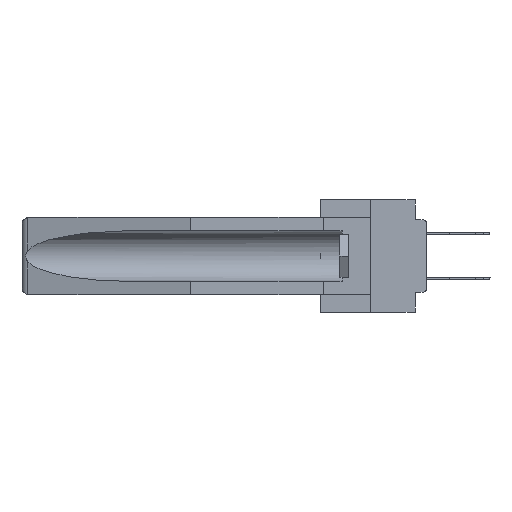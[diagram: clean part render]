
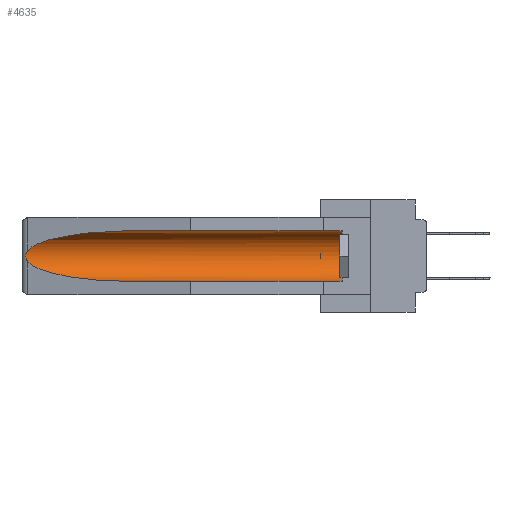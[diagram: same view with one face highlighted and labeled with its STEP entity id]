
A CAD part, left-side view. The second image highlights one B-rep face of the part: STEP entity #4635.
In plain terms, the highlighted cylindrical face has radius 2.857 mm (diameter 5.715 mm), a partial arc.
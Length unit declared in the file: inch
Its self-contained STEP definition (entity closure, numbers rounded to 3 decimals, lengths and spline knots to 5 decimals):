
#343 = VERTEX_POINT ( 'NONE', #15983 ) ;
#2285 = CARTESIAN_POINT ( 'NONE',  ( 0.25451, 1.48313, -0.09465 ) ) ;
#2305 = CARTESIAN_POINT ( 'NONE',  ( 0.155, 0.126, -0.059 ) ) ;
#3150 = CARTESIAN_POINT ( 'NONE',  ( 0.26654, 1.53092, -0.15636 ) ) ;
#3228 = CARTESIAN_POINT ( 'NONE',  ( 0.155, 1.07973, -0.059 ) ) ;
#3517 = VERTEX_POINT ( 'NONE', #33483 ) ;
#4357 = EDGE_LOOP ( 'NONE', ( #16851, #13182, #14924, #16887, #33822, #25248 ) ) ;
#4635 = ADVANCED_FACE ( 'NONE', ( #13232 ), #30506, .F. ) ;
#4799 = EDGE_CURVE ( 'NONE', #22760, #343, #28075, .T. ) ;
#6277 = CARTESIAN_POINT ( 'NONE',  ( 0.2675, 1.53308, -0.16763 ) ) ;
#8865 = DIRECTION ( 'NONE',  ( 0., 1., 0. ) ) ;
#9593 =( BOUNDED_CURVE ( )  B_SPLINE_CURVE ( 3, ( #3228, #29074, #2285, #34038 ),
 .UNSPECIFIED., .F., .F. ) 
 B_SPLINE_CURVE_WITH_KNOTS ( ( 4, 4 ),
 ( 4.71239, 6.08839 ),
 .UNSPECIFIED. ) 
 CURVE ( )  GEOMETRIC_REPRESENTATION_ITEM ( )  RATIONAL_B_SPLINE_CURVE ( ( 1., 0.848, 0.848, 1. ) ) 
 REPRESENTATION_ITEM ( '' )  );
#9688 = CARTESIAN_POINT ( 'NONE',  ( 0.26537, 1.52718, -0.14972 ) ) ;
#10539 = CARTESIAN_POINT ( 'NONE',  ( 0.26537, 1.52718, -0.14972 ) ) ;
#11886 =( BOUNDED_CURVE ( )  B_SPLINE_CURVE ( 3, ( #27432, #27709, #34202, #28121 ),
 .UNSPECIFIED., .F., .T. ) 
 B_SPLINE_CURVE_WITH_KNOTS ( ( 4, 4 ),
 ( 0.1948, 1.5708 ),
 .UNSPECIFIED. ) 
 CURVE ( )  GEOMETRIC_REPRESENTATION_ITEM ( )  RATIONAL_B_SPLINE_CURVE ( ( 1., 0.848, 0.848, 1. ) ) 
 REPRESENTATION_ITEM ( '' )  );
#12557 = CARTESIAN_POINT ( 'NONE',  ( 0.155, 0.126, -0.1715 ) ) ;
#13182 = ORIENTED_EDGE ( 'NONE', *, *, #37447, .T. ) ;
#13232 = FACE_OUTER_BOUND ( 'NONE', #4357, .T. ) ;
#13719 = LINE ( 'NONE', #17960, #37736 ) ;
#14924 = ORIENTED_EDGE ( 'NONE', *, *, #31422, .T. ) ;
#15839 = DIRECTION ( 'NONE',  ( 0., -1., 0. ) ) ;
#15983 = CARTESIAN_POINT ( 'NONE',  ( 0.155, 1.07973, -0.059 ) ) ;
#16851 = ORIENTED_EDGE ( 'NONE', *, *, #35183, .T. ) ;
#16887 = ORIENTED_EDGE ( 'NONE', *, *, #27997, .F. ) ;
#17960 = CARTESIAN_POINT ( 'NONE',  ( 0.155, -0.30754, -0.284 ) ) ;
#19195 = CARTESIAN_POINT ( 'NONE',  ( 0.26537, 1.52718, -0.19328 ) ) ;
#21794 = CARTESIAN_POINT ( 'NONE',  ( 0.155, -0.30754, -0.059 ) ) ;
#21871 = VERTEX_POINT ( 'NONE', #10539 ) ;
#22013 = CARTESIAN_POINT ( 'NONE',  ( 0.2673, 1.5327, -0.16383 ) ) ;
#22229 = VERTEX_POINT ( 'NONE', #28094 ) ;
#22760 = VERTEX_POINT ( 'NONE', #2305 ) ;
#23876 = AXIS2_PLACEMENT_3D ( 'NONE', #12557, #15839, #25237 ) ;
#24553 = EDGE_CURVE ( 'NONE', #3517, #22760, #28765, .T. ) ;
#25237 = DIRECTION ( 'NONE',  ( 0., 0., 1. ) ) ;
#25248 = ORIENTED_EDGE ( 'NONE', *, *, #4799, .T. ) ;
#27071 = VECTOR ( 'NONE', #30841, 39.37008 ) ;
#27432 = CARTESIAN_POINT ( 'NONE',  ( 0.26537, 1.52718, -0.19328 ) ) ;
#27709 = CARTESIAN_POINT ( 'NONE',  ( 0.25451, 1.48313, -0.24835 ) ) ;
#27997 = EDGE_CURVE ( 'NONE', #3517, #38197, #13719, .T. ) ;
#28007 = AXIS2_PLACEMENT_3D ( 'NONE', #30020, #36250, #33118 ) ;
#28075 = LINE ( 'NONE', #21794, #27071 ) ;
#28094 = CARTESIAN_POINT ( 'NONE',  ( 0.26537, 1.52718, -0.19328 ) ) ;
#28121 = CARTESIAN_POINT ( 'NONE',  ( 0.155, 1.07973, -0.284 ) ) ;
#28339 = CARTESIAN_POINT ( 'NONE',  ( 0.2673, 1.53269, -0.17917 ) ) ;
#28765 = CIRCLE ( 'NONE', #23876, 0.1125 ) ;
#29074 = CARTESIAN_POINT ( 'NONE',  ( 0.21114, 1.30732, -0.059 ) ) ;
#30020 = CARTESIAN_POINT ( 'NONE',  ( 0.155, -0.30754, -0.1715 ) ) ;
#30506 = CYLINDRICAL_SURFACE ( 'NONE', #28007, 0.1125 ) ;
#30841 = DIRECTION ( 'NONE',  ( 0., 1., 0. ) ) ;
#31422 = EDGE_CURVE ( 'NONE', #22229, #38197, #11886, .T. ) ;
#31550 = CARTESIAN_POINT ( 'NONE',  ( 0.26655, 1.53094, -0.18657 ) ) ;
#33118 = DIRECTION ( 'NONE',  ( 0., 0., 1. ) ) ;
#33265 = B_SPLINE_CURVE_WITH_KNOTS ( 'NONE', 3,
 ( #9688, #38052, #3150, #22013, #6277, #34788, #28339, #31550, #37928, #19195 ),
 .UNSPECIFIED., .F., .F.,
 ( 4, 2, 2, 2, 4 ),
 ( 0., 0.00029, 0.00058, 0.00087, 0.00117 ),
 .UNSPECIFIED. ) ;
#33483 = CARTESIAN_POINT ( 'NONE',  ( 0.155, 0.126, -0.284 ) ) ;
#33822 = ORIENTED_EDGE ( 'NONE', *, *, #24553, .T. ) ;
#34038 = CARTESIAN_POINT ( 'NONE',  ( 0.26537, 1.52718, -0.14972 ) ) ;
#34202 = CARTESIAN_POINT ( 'NONE',  ( 0.21114, 1.30732, -0.284 ) ) ;
#34788 = CARTESIAN_POINT ( 'NONE',  ( 0.2675, 1.53308, -0.17534 ) ) ;
#35183 = EDGE_CURVE ( 'NONE', #343, #21871, #9593, .T. ) ;
#36250 = DIRECTION ( 'NONE',  ( 0., 1., 0. ) ) ;
#37447 = EDGE_CURVE ( 'NONE', #21871, #22229, #33265, .T. ) ;
#37736 = VECTOR ( 'NONE', #8865, 39.37008 ) ;
#37928 = CARTESIAN_POINT ( 'NONE',  ( 0.26597, 1.5296, -0.19026 ) ) ;
#38052 = CARTESIAN_POINT ( 'NONE',  ( 0.26597, 1.52961, -0.15275 ) ) ;
#38197 = VERTEX_POINT ( 'NONE', #39245 ) ;
#39245 = CARTESIAN_POINT ( 'NONE',  ( 0.155, 1.07973, -0.284 ) ) ;
